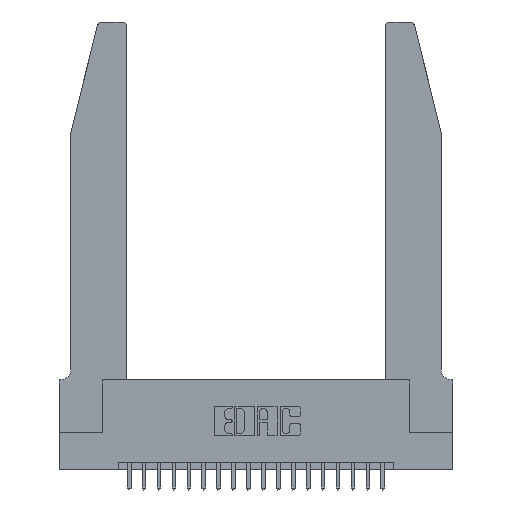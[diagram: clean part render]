
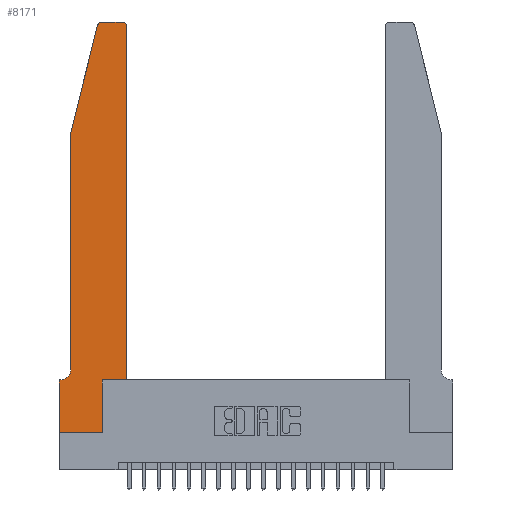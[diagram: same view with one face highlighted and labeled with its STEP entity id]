
A CAD part, top view. The second image highlights one B-rep face of the part: STEP entity #8171.
In plain terms, the highlighted planar face has unit normal (0, 0, 1).
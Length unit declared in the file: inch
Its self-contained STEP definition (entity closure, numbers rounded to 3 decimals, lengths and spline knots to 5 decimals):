
#100 = CARTESIAN_POINT ( 'NONE',  ( 0.4205, 2.75, 0.37 ) ) ;
#160 = DIRECTION ( 'NONE',  ( 1., 0., 0. ) ) ;
#561 = CARTESIAN_POINT ( 'NONE',  ( 0.2865, 0.35, 0.37 ) ) ;
#1018 = VERTEX_POINT ( 'NONE', #7516 ) ;
#1818 = CARTESIAN_POINT ( 'NONE',  ( 0.2605, 2.75, 0.37 ) ) ;
#2304 = DIRECTION ( 'NONE',  ( 1., 0., 0. ) ) ;
#2372 = LINE ( 'NONE', #10149, #17635 ) ;
#2517 = AXIS2_PLACEMENT_3D ( 'NONE', #16878, #10143, #13620 ) ;
#2877 = LINE ( 'NONE', #7386, #12812 ) ;
#2972 = EDGE_CURVE ( 'NONE', #13006, #3473, #8595, .T. ) ;
#3349 = VERTEX_POINT ( 'NONE', #16476 ) ;
#3473 = VERTEX_POINT ( 'NONE', #14637 ) ;
#3619 = CARTESIAN_POINT ( 'NONE',  ( 0.0755, 2., 0.37 ) ) ;
#3658 = ORIENTED_EDGE ( 'NONE', *, *, #21466, .T. ) ;
#3686 = DIRECTION ( 'NONE',  ( 0., 0., 1. ) ) ;
#3837 = DIRECTION ( 'NONE',  ( 1., 0., 0. ) ) ;
#3981 = DIRECTION ( 'NONE',  ( -0.239, -0.971, 0. ) ) ;
#4062 = CARTESIAN_POINT ( 'NONE',  ( 0.0755, 0.42, 0.37 ) ) ;
#4078 = EDGE_CURVE ( 'NONE', #21632, #16626, #14592, .T. ) ;
#4108 = LINE ( 'NONE', #18601, #4674 ) ;
#4153 = VECTOR ( 'NONE', #16150, 39.37008 ) ;
#4190 = VECTOR ( 'NONE', #15680, 39.37008 ) ;
#4222 = CARTESIAN_POINT ( 'NONE',  ( 0., 0., 0.37 ) ) ;
#4526 = EDGE_CURVE ( 'NONE', #16626, #14464, #8736, .T. ) ;
#4674 = VECTOR ( 'NONE', #160, 39.37008 ) ;
#5505 = CARTESIAN_POINT ( 'NONE',  ( 0.4205, 2.72, 0.37 ) ) ;
#5674 = ORIENTED_EDGE ( 'NONE', *, *, #2972, .T. ) ;
#6936 = VECTOR ( 'NONE', #13664, 39.37008 ) ;
#7164 = AXIS2_PLACEMENT_3D ( 'NONE', #5505, #7319, #2304 ) ;
#7319 = DIRECTION ( 'NONE',  ( 0., 0., 1. ) ) ;
#7386 = CARTESIAN_POINT ( 'NONE',  ( 0.0755, 2., 0.37 ) ) ;
#7516 = CARTESIAN_POINT ( 'NONE',  ( 0.2865, 0., 0.37 ) ) ;
#7761 = FACE_OUTER_BOUND ( 'NONE', #17420, .T. ) ;
#7961 = VERTEX_POINT ( 'NONE', #16359 ) ;
#8171 = ADVANCED_FACE ( 'NONE', ( #7761 ), #17424, .T. ) ;
#8274 = VERTEX_POINT ( 'NONE', #561 ) ;
#8301 = EDGE_CURVE ( 'NONE', #3473, #7961, #2877, .T. ) ;
#8595 = CIRCLE ( 'NONE', #2517, 0.03 ) ;
#8627 = CARTESIAN_POINT ( 'NONE',  ( 0.4505, 0.35, 0.37 ) ) ;
#8661 = EDGE_CURVE ( 'NONE', #1018, #8274, #21544, .T. ) ;
#8736 = LINE ( 'NONE', #4222, #4153 ) ;
#8749 = ORIENTED_EDGE ( 'NONE', *, *, #16480, .T. ) ;
#8852 = ORIENTED_EDGE ( 'NONE', *, *, #19408, .T. ) ;
#9180 = DIRECTION ( 'NONE',  ( 0., 0., -1. ) ) ;
#9927 = LINE ( 'NONE', #1818, #22130 ) ;
#9979 = EDGE_CURVE ( 'NONE', #14464, #1018, #4108, .T. ) ;
#10143 = DIRECTION ( 'NONE',  ( 0., 0., 1. ) ) ;
#10149 = CARTESIAN_POINT ( 'NONE',  ( 0.4505, 0.35, 0.37 ) ) ;
#10971 = CARTESIAN_POINT ( 'NONE',  ( 0.0055, 0.42, 0.37 ) ) ;
#11015 = ORIENTED_EDGE ( 'NONE', *, *, #9979, .T. ) ;
#11131 = ORIENTED_EDGE ( 'NONE', *, *, #13116, .T. ) ;
#11223 = LINE ( 'NONE', #3619, #6936 ) ;
#11332 = VERTEX_POINT ( 'NONE', #18428 ) ;
#11868 = DIRECTION ( 'NONE',  ( 0., 1., 0. ) ) ;
#12012 = LINE ( 'NONE', #8627, #4190 ) ;
#12411 = DIRECTION ( 'NONE',  ( -1., 0., 0. ) ) ;
#12470 = EDGE_CURVE ( 'NONE', #11332, #3349, #2372, .T. ) ;
#12812 = VECTOR ( 'NONE', #3981, 39.37008 ) ;
#12858 = DIRECTION ( 'NONE',  ( -1., 0., 0. ) ) ;
#13006 = VERTEX_POINT ( 'NONE', #20498 ) ;
#13116 = EDGE_CURVE ( 'NONE', #14094, #13006, #9927, .T. ) ;
#13139 = CARTESIAN_POINT ( 'NONE',  ( 0., 0., 0.37 ) ) ;
#13620 = DIRECTION ( 'NONE',  ( 1., 0., 0. ) ) ;
#13664 = DIRECTION ( 'NONE',  ( 0., -1., 0. ) ) ;
#13754 = DIRECTION ( 'NONE',  ( 0., 1., 0. ) ) ;
#13987 = ORIENTED_EDGE ( 'NONE', *, *, #16481, .T. ) ;
#14044 = CARTESIAN_POINT ( 'NONE',  ( 0., 0.35, 0.37 ) ) ;
#14094 = VERTEX_POINT ( 'NONE', #100 ) ;
#14464 = VERTEX_POINT ( 'NONE', #13139 ) ;
#14592 = LINE ( 'NONE', #14856, #20716 ) ;
#14637 = CARTESIAN_POINT ( 'NONE',  ( 0.25487, 2.72718, 0.37 ) ) ;
#14856 = CARTESIAN_POINT ( 'NONE',  ( 0.0755, 0.35, 0.37 ) ) ;
#15220 = AXIS2_PLACEMENT_3D ( 'NONE', #14044, #3686, #3837 ) ;
#15680 = DIRECTION ( 'NONE',  ( 1., 0., 0. ) ) ;
#15836 = ORIENTED_EDGE ( 'NONE', *, *, #8661, .T. ) ;
#16016 = CARTESIAN_POINT ( 'NONE',  ( 0.0055, 0.35, 0.37 ) ) ;
#16150 = DIRECTION ( 'NONE',  ( 0., -1., 0. ) ) ;
#16352 = CARTESIAN_POINT ( 'NONE',  ( 0., 0.35, 0.37 ) ) ;
#16359 = CARTESIAN_POINT ( 'NONE',  ( 0.0755, 2., 0.37 ) ) ;
#16476 = CARTESIAN_POINT ( 'NONE',  ( 0.4505, 2.72, 0.37 ) ) ;
#16480 = EDGE_CURVE ( 'NONE', #16522, #21632, #20921, .T. ) ;
#16481 = EDGE_CURVE ( 'NONE', #3349, #14094, #20129, .T. ) ;
#16522 = VERTEX_POINT ( 'NONE', #4062 ) ;
#16625 = ORIENTED_EDGE ( 'NONE', *, *, #12470, .T. ) ;
#16626 = VERTEX_POINT ( 'NONE', #16352 ) ;
#16878 = CARTESIAN_POINT ( 'NONE',  ( 0.284, 2.72, 0.37 ) ) ;
#17236 = DIRECTION ( 'NONE',  ( -1., 0., 0. ) ) ;
#17420 = EDGE_LOOP ( 'NONE', ( #11131, #5674, #17672, #8852, #8749, #17888, #17729, #11015, #15836, #3658, #16625, #13987 ) ) ;
#17424 = PLANE ( 'NONE',  #15220 ) ;
#17547 = AXIS2_PLACEMENT_3D ( 'NONE', #10971, #9180, #12411 ) ;
#17635 = VECTOR ( 'NONE', #11868, 39.37008 ) ;
#17672 = ORIENTED_EDGE ( 'NONE', *, *, #8301, .T. ) ;
#17729 = ORIENTED_EDGE ( 'NONE', *, *, #4526, .T. ) ;
#17888 = ORIENTED_EDGE ( 'NONE', *, *, #4078, .T. ) ;
#18428 = CARTESIAN_POINT ( 'NONE',  ( 0.4505, 0.35, 0.37 ) ) ;
#18601 = CARTESIAN_POINT ( 'NONE',  ( 0., 0., 0.37 ) ) ;
#19408 = EDGE_CURVE ( 'NONE', #7961, #16522, #11223, .T. ) ;
#19950 = VECTOR ( 'NONE', #13754, 39.37008 ) ;
#20129 = CIRCLE ( 'NONE', #7164, 0.03 ) ;
#20282 = CARTESIAN_POINT ( 'NONE',  ( 0.2865, 0.35, 0.37 ) ) ;
#20498 = CARTESIAN_POINT ( 'NONE',  ( 0.284, 2.75, 0.37 ) ) ;
#20716 = VECTOR ( 'NONE', #12858, 39.37008 ) ;
#20921 = CIRCLE ( 'NONE', #17547, 0.07 ) ;
#21466 = EDGE_CURVE ( 'NONE', #8274, #11332, #12012, .T. ) ;
#21544 = LINE ( 'NONE', #20282, #19950 ) ;
#21632 = VERTEX_POINT ( 'NONE', #16016 ) ;
#22130 = VECTOR ( 'NONE', #17236, 39.37008 ) ;
